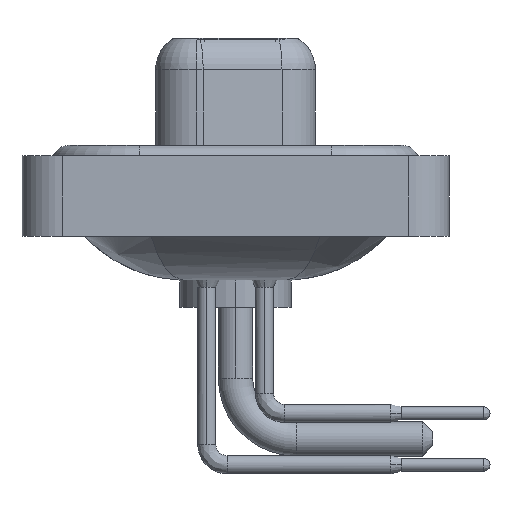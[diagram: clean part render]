
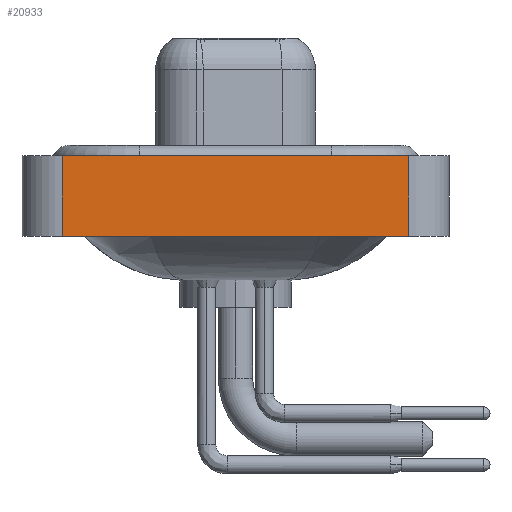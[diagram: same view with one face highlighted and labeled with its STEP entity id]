
A CAD part, left-side view. The second image highlights one B-rep face of the part: STEP entity #20933.
In plain terms, the highlighted planar face has unit normal (-1, 0, 0).
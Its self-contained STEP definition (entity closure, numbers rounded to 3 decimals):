
#1387 = CARTESIAN_POINT ( 'NONE',  ( -7.3, -8.55, -3.6 ) ) ;
#1920 = CARTESIAN_POINT ( 'NONE',  ( -7.3, -8.55, -3.6 ) ) ;
#4078 = EDGE_LOOP ( 'NONE', ( #8861, #13611, #19402, #21842 ) ) ;
#4442 = DIRECTION ( 'NONE',  ( 0., 0., 1. ) ) ;
#4572 = DIRECTION ( 'NONE',  ( 0., -1., 0. ) ) ;
#5423 = CARTESIAN_POINT ( 'NONE',  ( -7.3, -8.55, 0.4 ) ) ;
#6135 = DIRECTION ( 'NONE',  ( -1., 0., 0. ) ) ;
#6811 = CARTESIAN_POINT ( 'NONE',  ( -7.3, -8.55, 0.4 ) ) ;
#7035 = EDGE_CURVE ( 'NONE', #13214, #13237, #19282, .T. ) ;
#8298 = EDGE_CURVE ( 'NONE', #16664, #13237, #19457, .T. ) ;
#8507 = CARTESIAN_POINT ( 'NONE',  ( -7.3, 8.55, -3.6 ) ) ;
#8707 = VECTOR ( 'NONE', #19395, 1000. ) ;
#8861 = ORIENTED_EDGE ( 'NONE', *, *, #7035, .T. ) ;
#9306 = PLANE ( 'NONE',  #18192 ) ;
#9383 = VECTOR ( 'NONE', #10984, 1000. ) ;
#10970 = VECTOR ( 'NONE', #4572, 1000. ) ;
#10984 = DIRECTION ( 'NONE',  ( 0., -1., 0. ) ) ;
#11040 = CARTESIAN_POINT ( 'NONE',  ( -7.3, 8.55, -3.6 ) ) ;
#11129 = CARTESIAN_POINT ( 'NONE',  ( -7.3, -8.55, -3.6 ) ) ;
#13039 = FACE_OUTER_BOUND ( 'NONE', #4078, .T. ) ;
#13214 = VERTEX_POINT ( 'NONE', #1920 ) ;
#13237 = VERTEX_POINT ( 'NONE', #6811 ) ;
#13611 = ORIENTED_EDGE ( 'NONE', *, *, #8298, .F. ) ;
#15542 = EDGE_CURVE ( 'NONE', #18458, #16664, #16215, .T. ) ;
#15881 = CARTESIAN_POINT ( 'NONE',  ( -7.3, -8.55, -3.6 ) ) ;
#16215 = LINE ( 'NONE', #11040, #22063 ) ;
#16664 = VERTEX_POINT ( 'NONE', #20183 ) ;
#17088 = EDGE_CURVE ( 'NONE', #18458, #13214, #20161, .T. ) ;
#18192 = AXIS2_PLACEMENT_3D ( 'NONE', #11129, #6135, #4442 ) ;
#18458 = VERTEX_POINT ( 'NONE', #8507 ) ;
#19282 = LINE ( 'NONE', #15881, #8707 ) ;
#19287 = DIRECTION ( 'NONE',  ( 0., 0., 1. ) ) ;
#19395 = DIRECTION ( 'NONE',  ( 0., 0., 1. ) ) ;
#19402 = ORIENTED_EDGE ( 'NONE', *, *, #15542, .F. ) ;
#19457 = LINE ( 'NONE', #5423, #9383 ) ;
#20161 = LINE ( 'NONE', #1387, #10970 ) ;
#20183 = CARTESIAN_POINT ( 'NONE',  ( -7.3, 8.55, 0.4 ) ) ;
#20933 = ADVANCED_FACE ( 'NONE', ( #13039 ), #9306, .T. ) ;
#21842 = ORIENTED_EDGE ( 'NONE', *, *, #17088, .T. ) ;
#22063 = VECTOR ( 'NONE', #19287, 1000. ) ;
